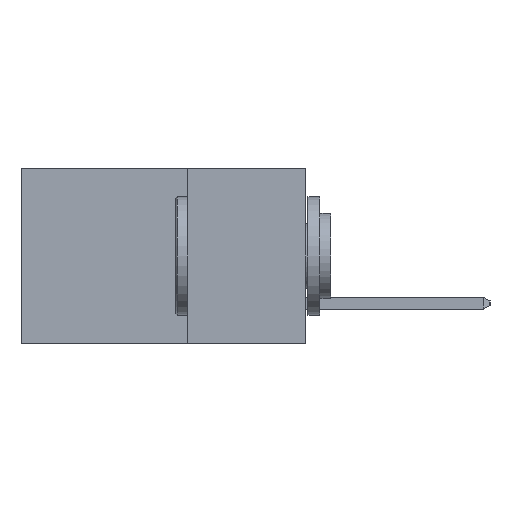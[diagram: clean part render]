
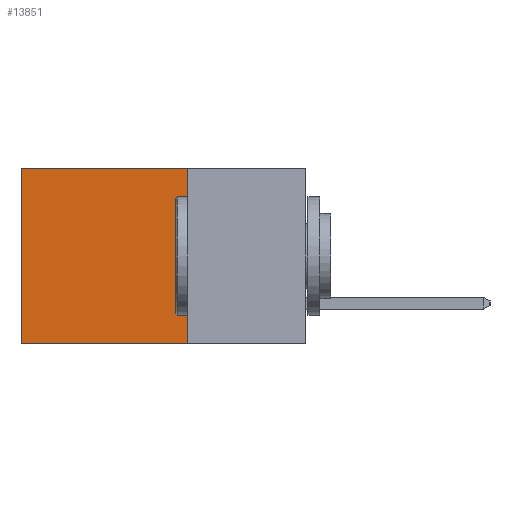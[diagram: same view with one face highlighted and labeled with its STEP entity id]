
A CAD part, left-side view. The second image highlights one B-rep face of the part: STEP entity #13851.
In plain terms, the highlighted planar face has unit normal (-1, 0, 0).
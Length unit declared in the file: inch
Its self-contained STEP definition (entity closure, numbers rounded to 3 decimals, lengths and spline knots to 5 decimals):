
#231 = ORIENTED_EDGE ( 'NONE', *, *, #1088, .F. ) ;
#332 = LINE ( 'NONE', #14636, #9643 ) ;
#561 = VERTEX_POINT ( 'NONE', #9204 ) ;
#884 = EDGE_CURVE ( 'NONE', #3085, #561, #12138, .T. ) ;
#981 = VECTOR ( 'NONE', #7489, 39.37008 ) ;
#1088 = EDGE_CURVE ( 'NONE', #561, #1422, #332, .T. ) ;
#1422 = VERTEX_POINT ( 'NONE', #10166 ) ;
#2071 = DIRECTION ( 'NONE',  ( 1., 0., 0. ) ) ;
#2077 = LINE ( 'NONE', #6127, #14177 ) ;
#2125 = DIRECTION ( 'NONE',  ( 0., 1., 0. ) ) ;
#2731 = ORIENTED_EDGE ( 'NONE', *, *, #12631, .T. ) ;
#3085 = VERTEX_POINT ( 'NONE', #12873 ) ;
#3959 = VECTOR ( 'NONE', #9086, 39.37008 ) ;
#4237 = VERTEX_POINT ( 'NONE', #11250 ) ;
#4574 = ORIENTED_EDGE ( 'NONE', *, *, #884, .F. ) ;
#4838 = EDGE_LOOP ( 'NONE', ( #8556, #231, #4574, #2731 ) ) ;
#6127 = CARTESIAN_POINT ( 'NONE',  ( 0.298, 0.25, 0. ) ) ;
#6412 = AXIS2_PLACEMENT_3D ( 'NONE', #6865, #2071, #10398 ) ;
#6810 = FACE_OUTER_BOUND ( 'NONE', #4838, .T. ) ;
#6865 = CARTESIAN_POINT ( 'NONE',  ( 0.298, 0.25, 0. ) ) ;
#7417 = CARTESIAN_POINT ( 'NONE',  ( 0.298, 0.6, 0. ) ) ;
#7489 = DIRECTION ( 'NONE',  ( 0., 0., -1. ) ) ;
#7503 = EDGE_CURVE ( 'NONE', #4237, #1422, #13564, .T. ) ;
#8556 = ORIENTED_EDGE ( 'NONE', *, *, #7503, .T. ) ;
#9086 = DIRECTION ( 'NONE',  ( 0., 0., -1. ) ) ;
#9204 = CARTESIAN_POINT ( 'NONE',  ( 0.298, 0.25, -0.37 ) ) ;
#9247 = PLANE ( 'NONE',  #6412 ) ;
#9643 = VECTOR ( 'NONE', #2125, 39.37008 ) ;
#10166 = CARTESIAN_POINT ( 'NONE',  ( 0.298, 0.6, -0.37 ) ) ;
#10398 = DIRECTION ( 'NONE',  ( 0., 0., -1. ) ) ;
#11250 = CARTESIAN_POINT ( 'NONE',  ( 0.298, 0.6, 0. ) ) ;
#12138 = LINE ( 'NONE', #14100, #3959 ) ;
#12631 = EDGE_CURVE ( 'NONE', #3085, #4237, #2077, .T. ) ;
#12873 = CARTESIAN_POINT ( 'NONE',  ( 0.298, 0.25, 0. ) ) ;
#13564 = LINE ( 'NONE', #7417, #981 ) ;
#13851 = ADVANCED_FACE ( 'NONE', ( #6810 ), #9247, .F. ) ;
#14100 = CARTESIAN_POINT ( 'NONE',  ( 0.298, 0.25, 0. ) ) ;
#14177 = VECTOR ( 'NONE', #15328, 39.37008 ) ;
#14636 = CARTESIAN_POINT ( 'NONE',  ( 0.298, 0.25, -0.37 ) ) ;
#15328 = DIRECTION ( 'NONE',  ( 0., 1., 0. ) ) ;
